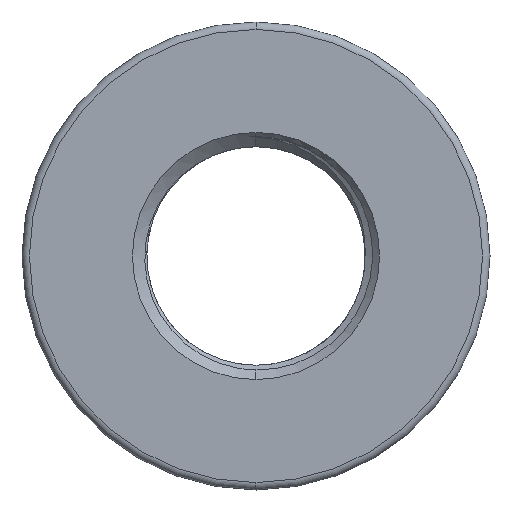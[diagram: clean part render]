
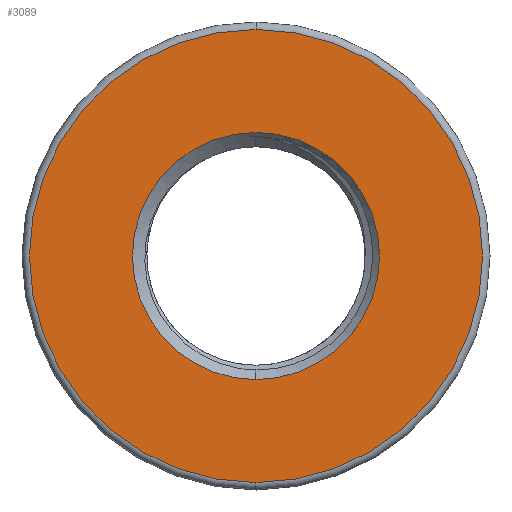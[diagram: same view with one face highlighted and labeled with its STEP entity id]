
A CAD part, left-side view. The second image highlights one B-rep face of the part: STEP entity #3089.
In plain terms, the highlighted planar face has unit normal (-1, 0, 0).
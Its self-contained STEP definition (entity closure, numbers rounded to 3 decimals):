
#18 = AXIS2_PLACEMENT_3D ( 'NONE', #2534, #529, #2887 ) ;
#59 = CARTESIAN_POINT ( 'NONE',  ( 0., 0., 0. ) ) ;
#119 = VERTEX_POINT ( 'NONE', #2663 ) ;
#291 = DIRECTION ( 'NONE',  ( 1., 0., 0. ) ) ;
#349 = ORIENTED_EDGE ( 'NONE', *, *, #2653, .T. ) ;
#383 = EDGE_CURVE ( 'NONE', #3495, #119, #2521, .T. ) ;
#394 = DIRECTION ( 'NONE',  ( 0., 0., 1. ) ) ;
#410 = CIRCLE ( 'NONE', #3474, 12.049 ) ;
#485 = CARTESIAN_POINT ( 'NONE',  ( 0., 0., 0. ) ) ;
#529 = DIRECTION ( 'NONE',  ( 1., 0., 0. ) ) ;
#663 = FACE_BOUND ( 'NONE', #3570, .T. ) ;
#821 = DIRECTION ( 'NONE',  ( 0., 0., 1. ) ) ;
#1014 = ORIENTED_EDGE ( 'NONE', *, *, #3677, .T. ) ;
#1298 = CARTESIAN_POINT ( 'NONE',  ( 0., 0., -6.571 ) ) ;
#1309 = CIRCLE ( 'NONE', #3049, 12.049 ) ;
#1325 = CARTESIAN_POINT ( 'NONE',  ( 0., 0., 0. ) ) ;
#1463 = EDGE_LOOP ( 'NONE', ( #2257, #1014 ) ) ;
#1629 = PLANE ( 'NONE',  #4100 ) ;
#1925 = AXIS2_PLACEMENT_3D ( 'NONE', #2304, #291, #2641 ) ;
#1985 = DIRECTION ( 'NONE',  ( -1., 0., 0. ) ) ;
#2257 = ORIENTED_EDGE ( 'NONE', *, *, #2758, .T. ) ;
#2304 = CARTESIAN_POINT ( 'NONE',  ( 0., 0., 0. ) ) ;
#2395 = DIRECTION ( 'NONE',  ( -1., 0., 0. ) ) ;
#2521 = CIRCLE ( 'NONE', #18, 6.571 ) ;
#2534 = CARTESIAN_POINT ( 'NONE',  ( 0., 0., 0. ) ) ;
#2641 = DIRECTION ( 'NONE',  ( 0., 0., 1. ) ) ;
#2653 = EDGE_CURVE ( 'NONE', #119, #3495, #4011, .T. ) ;
#2663 = CARTESIAN_POINT ( 'NONE',  ( 0., 0., 6.571 ) ) ;
#2758 = EDGE_CURVE ( 'NONE', #3732, #3846, #1309, .T. ) ;
#2839 = DIRECTION ( 'NONE',  ( -1., 0., 0. ) ) ;
#2855 = ORIENTED_EDGE ( 'NONE', *, *, #383, .T. ) ;
#2887 = DIRECTION ( 'NONE',  ( 0., 0., 1. ) ) ;
#3049 = AXIS2_PLACEMENT_3D ( 'NONE', #59, #2395, #394 ) ;
#3089 = ADVANCED_FACE ( 'NONE', ( #663, #3156 ), #1629, .T. ) ;
#3156 = FACE_OUTER_BOUND ( 'NONE', #1463, .T. ) ;
#3246 = CARTESIAN_POINT ( 'NONE',  ( 0., 0., -12.049 ) ) ;
#3474 = AXIS2_PLACEMENT_3D ( 'NONE', #485, #2839, #821 ) ;
#3495 = VERTEX_POINT ( 'NONE', #1298 ) ;
#3570 = EDGE_LOOP ( 'NONE', ( #349, #2855 ) ) ;
#3677 = EDGE_CURVE ( 'NONE', #3846, #3732, #410, .T. ) ;
#3732 = VERTEX_POINT ( 'NONE', #4216 ) ;
#3846 = VERTEX_POINT ( 'NONE', #3246 ) ;
#4011 = CIRCLE ( 'NONE', #1925, 6.571 ) ;
#4100 = AXIS2_PLACEMENT_3D ( 'NONE', #1325, #1985, #4363 ) ;
#4216 = CARTESIAN_POINT ( 'NONE',  ( 0., 0., 12.049 ) ) ;
#4363 = DIRECTION ( 'NONE',  ( 0., 0., 1. ) ) ;
